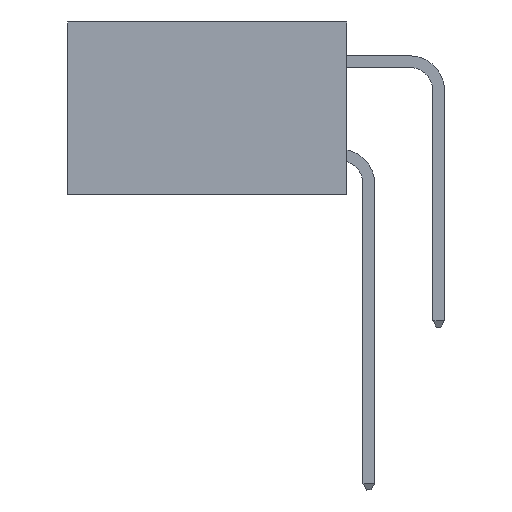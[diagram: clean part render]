
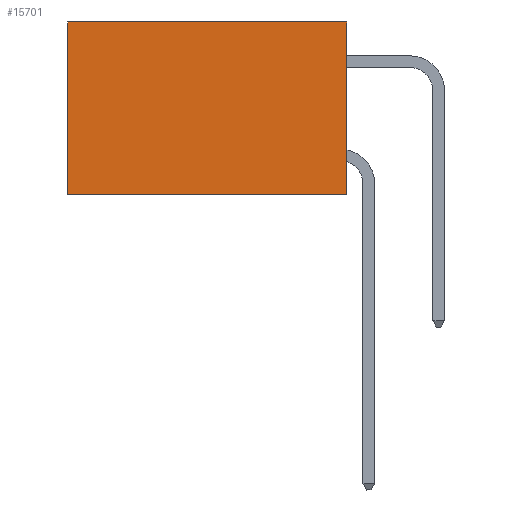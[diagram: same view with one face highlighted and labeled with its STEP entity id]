
A CAD part, left-side view. The second image highlights one B-rep face of the part: STEP entity #15701.
In plain terms, the highlighted planar face has unit normal (-1, 0, 0).
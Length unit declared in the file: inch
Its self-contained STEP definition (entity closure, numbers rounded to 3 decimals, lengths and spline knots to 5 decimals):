
#497 = CARTESIAN_POINT ( 'NONE',  ( 0.2875, 0., 0. ) ) ;
#1319 = LINE ( 'NONE', #14302, #13457 ) ;
#1656 = EDGE_CURVE ( 'NONE', #8586, #10388, #2784, .T. ) ;
#2273 = CARTESIAN_POINT ( 'NONE',  ( 0.2875, 0., 0. ) ) ;
#2784 = LINE ( 'NONE', #7959, #24464 ) ;
#4948 = DIRECTION ( 'NONE',  ( 0., 0., -1. ) ) ;
#5101 = FACE_OUTER_BOUND ( 'NONE', #10075, .T. ) ;
#6334 = ORIENTED_EDGE ( 'NONE', *, *, #7999, .T. ) ;
#6596 = CARTESIAN_POINT ( 'NONE',  ( 0.2875, 0., -0.37 ) ) ;
#7397 = EDGE_CURVE ( 'NONE', #15911, #10824, #19775, .T. ) ;
#7959 = CARTESIAN_POINT ( 'NONE',  ( 0.2875, 0., 0. ) ) ;
#7999 = EDGE_CURVE ( 'NONE', #10388, #10824, #1319, .T. ) ;
#8001 = DIRECTION ( 'NONE',  ( 0., 0., -1. ) ) ;
#8586 = VERTEX_POINT ( 'NONE', #14775 ) ;
#8834 = ORIENTED_EDGE ( 'NONE', *, *, #15540, .F. ) ;
#10075 = EDGE_LOOP ( 'NONE', ( #6334, #21525, #8834, #18901 ) ) ;
#10388 = VERTEX_POINT ( 'NONE', #17634 ) ;
#10447 = LINE ( 'NONE', #497, #11334 ) ;
#10810 = DIRECTION ( 'NONE',  ( 0., 1., 0. ) ) ;
#10824 = VERTEX_POINT ( 'NONE', #19195 ) ;
#11334 = VECTOR ( 'NONE', #11950, 39.37008 ) ;
#11950 = DIRECTION ( 'NONE',  ( 0., 0., -1. ) ) ;
#13457 = VECTOR ( 'NONE', #4948, 39.37008 ) ;
#13587 = DIRECTION ( 'NONE',  ( 0., 1., 0. ) ) ;
#13630 = PLANE ( 'NONE',  #15373 ) ;
#14302 = CARTESIAN_POINT ( 'NONE',  ( 0.2875, 0.6, 0. ) ) ;
#14775 = CARTESIAN_POINT ( 'NONE',  ( 0.2875, 0., 0. ) ) ;
#15373 = AXIS2_PLACEMENT_3D ( 'NONE', #2273, #17483, #8001 ) ;
#15540 = EDGE_CURVE ( 'NONE', #8586, #15911, #10447, .T. ) ;
#15701 = ADVANCED_FACE ( 'NONE', ( #5101 ), #13630, .F. ) ;
#15911 = VERTEX_POINT ( 'NONE', #19132 ) ;
#17483 = DIRECTION ( 'NONE',  ( 1., 0., 0. ) ) ;
#17634 = CARTESIAN_POINT ( 'NONE',  ( 0.2875, 0.6, 0. ) ) ;
#18901 = ORIENTED_EDGE ( 'NONE', *, *, #1656, .T. ) ;
#19132 = CARTESIAN_POINT ( 'NONE',  ( 0.2875, 0., -0.37 ) ) ;
#19195 = CARTESIAN_POINT ( 'NONE',  ( 0.2875, 0.6, -0.37 ) ) ;
#19775 = LINE ( 'NONE', #6596, #24218 ) ;
#21525 = ORIENTED_EDGE ( 'NONE', *, *, #7397, .F. ) ;
#24218 = VECTOR ( 'NONE', #10810, 39.37008 ) ;
#24464 = VECTOR ( 'NONE', #13587, 39.37008 ) ;
